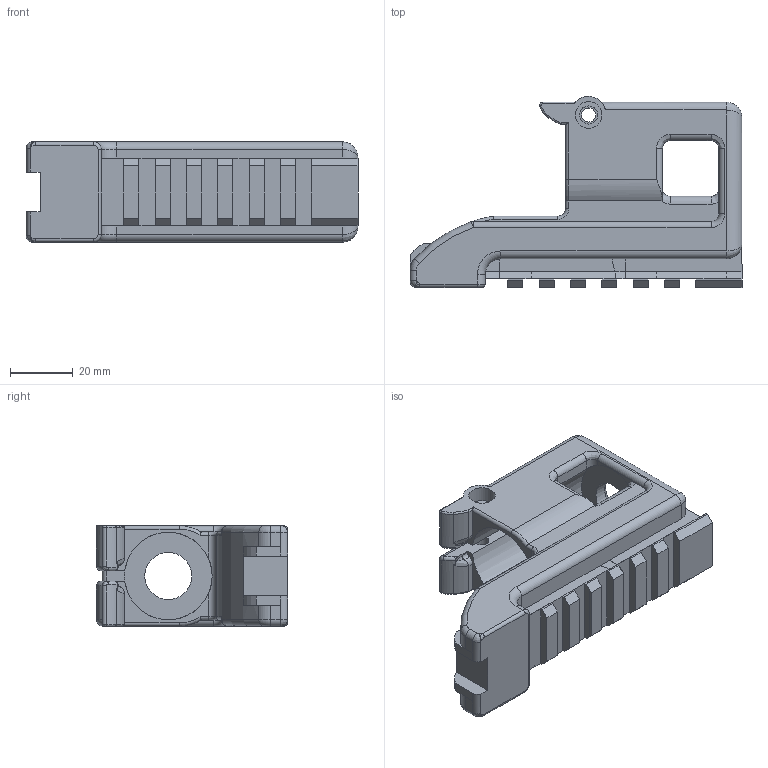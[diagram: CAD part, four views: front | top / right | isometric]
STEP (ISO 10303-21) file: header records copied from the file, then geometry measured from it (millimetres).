
FILE_DESCRIPTION(/* description */ (''),/* implementation_level */ '2;1');
FILE_NAME(/* name */ 'vz61 Handguard.step',/* time_stamp */ '2021-02-09T08:46:27-07:00',/* author */ (''),/* organization */ (''),/* preprocessor_version */ 'ST-DEVELOPER v18.1',/* originating_system */ 'Autodesk Translation Framework v9.7.1.1290',/* authorisation */ '');
FILE_SCHEMA (('AUTOMOTIVE_DESIGN { 1 0 10303 214 3 1 1 }'));
Length unit declared in the file: millimetre
Products named in the file (1): vz61 Handguard
Bounding box: 106 x 60.99 x 32 mm (x, y, z)
Volume: 87916.3 mm3; surface area: 23838.4 mm2
Topology: 1 solids, 1 shells, 344 faces, 912 edges, 561 vertices
Faces by surface type: plane 197, cylinder 83, bspline 36, torus 27, cone 1
Full cylindrical faces by diameter (mm): 4.5 x1, 5.8 x1, 8.5 x1, 15 x1, 28 x1
Entity records: 11702 total; most frequent: CARTESIAN_POINT 3334, ORIENTED_EDGE 1808, DIRECTION 1637, EDGE_CURVE 904, LINE 601, VECTOR 601, VERTEX_POINT 561, AXIS2_PLACEMENT_3D 518
